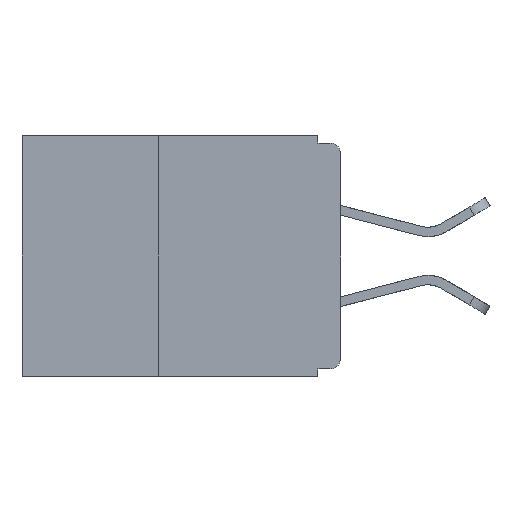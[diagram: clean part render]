
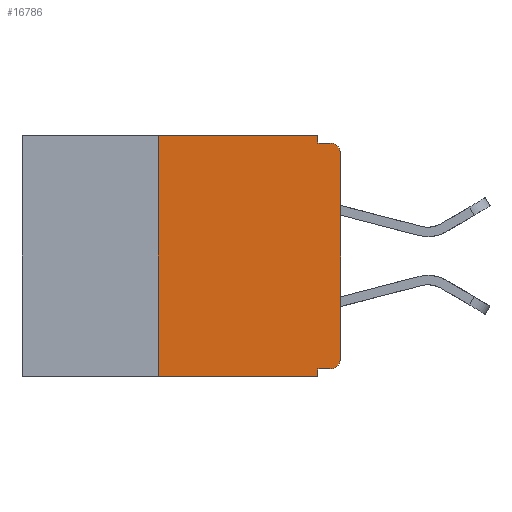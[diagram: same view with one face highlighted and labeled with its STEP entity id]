
A CAD part, left-side view. The second image highlights one B-rep face of the part: STEP entity #16786.
In plain terms, the highlighted planar face has unit normal (-1, 0, 0).
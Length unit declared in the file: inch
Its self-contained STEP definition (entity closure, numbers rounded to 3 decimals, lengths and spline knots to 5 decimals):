
#333 = EDGE_CURVE ( 'NONE', #7739, #5387, #16502, .T. ) ;
#369 = EDGE_CURVE ( 'NONE', #20299, #21853, #20265, .T. ) ;
#513 = ORIENTED_EDGE ( 'NONE', *, *, #4288, .T. ) ;
#768 = EDGE_CURVE ( 'NONE', #16155, #20713, #16186, .T. ) ;
#907 = FACE_OUTER_BOUND ( 'NONE', #26456, .T. ) ;
#1850 = EDGE_CURVE ( 'NONE', #24167, #23509, #6395, .T. ) ;
#2306 = LINE ( 'NONE', #22788, #8103 ) ;
#2898 = ORIENTED_EDGE ( 'NONE', *, *, #369, .F. ) ;
#3325 = AXIS2_PLACEMENT_3D ( 'NONE', #27504, #6271, #21327 ) ;
#3384 = VERTEX_POINT ( 'NONE', #24861 ) ;
#3418 = VECTOR ( 'NONE', #6739, 39.37008 ) ;
#3450 = EDGE_CURVE ( 'NONE', #23509, #7739, #2306, .T. ) ;
#4116 = CARTESIAN_POINT ( 'NONE',  ( 0., 0.031, 0. ) ) ;
#4288 = EDGE_CURVE ( 'NONE', #16155, #3384, #4691, .T. ) ;
#4626 = ORIENTED_EDGE ( 'NONE', *, *, #19297, .F. ) ;
#4691 = LINE ( 'NONE', #25082, #14783 ) ;
#4969 = LINE ( 'NONE', #11244, #21479 ) ;
#5387 = VERTEX_POINT ( 'NONE', #11502 ) ;
#6271 = DIRECTION ( 'NONE',  ( 1., 0., 0. ) ) ;
#6303 = CARTESIAN_POINT ( 'NONE',  ( 0., 0.25, -0.33 ) ) ;
#6395 = CIRCLE ( 'NONE', #24870, 0.015 ) ;
#6739 = DIRECTION ( 'NONE',  ( 0., 0., -1. ) ) ;
#7111 = EDGE_CURVE ( 'NONE', #21853, #5387, #20381, .T. ) ;
#7495 = CARTESIAN_POINT ( 'NONE',  ( 0., 0.25, -0.33 ) ) ;
#7684 = DIRECTION ( 'NONE',  ( -1., 0., 0. ) ) ;
#7739 = VERTEX_POINT ( 'NONE', #9589 ) ;
#7931 = CARTESIAN_POINT ( 'NONE',  ( 0., 0.015, -0.305 ) ) ;
#8103 = VECTOR ( 'NONE', #22433, 39.37008 ) ;
#8962 = VECTOR ( 'NONE', #20363, 39.37008 ) ;
#9033 = DIRECTION ( 'NONE',  ( 0., 0., -1. ) ) ;
#9088 = CARTESIAN_POINT ( 'NONE',  ( 0., 0.015, -0.32 ) ) ;
#9246 = EDGE_CURVE ( 'NONE', #26113, #3384, #22892, .T. ) ;
#9589 = CARTESIAN_POINT ( 'NONE',  ( 0., 0., -0.025 ) ) ;
#9599 = DIRECTION ( 'NONE',  ( 0., 1., 0. ) ) ;
#10037 = ORIENTED_EDGE ( 'NONE', *, *, #768, .F. ) ;
#10521 = DIRECTION ( 'NONE',  ( 0., 0., 1. ) ) ;
#11244 = CARTESIAN_POINT ( 'NONE',  ( 0., 0.437, 0. ) ) ;
#11502 = CARTESIAN_POINT ( 'NONE',  ( 0., 0.015, -0.01 ) ) ;
#11732 = ORIENTED_EDGE ( 'NONE', *, *, #333, .T. ) ;
#12503 = CARTESIAN_POINT ( 'NONE',  ( 0., 0.031, -0.33 ) ) ;
#12570 = DIRECTION ( 'NONE',  ( 0., 0., -1. ) ) ;
#12828 = CARTESIAN_POINT ( 'NONE',  ( 0., 0.031, -0.32 ) ) ;
#14371 = ORIENTED_EDGE ( 'NONE', *, *, #24363, .F. ) ;
#14783 = VECTOR ( 'NONE', #25294, 39.37008 ) ;
#15270 = VECTOR ( 'NONE', #9599, 39.37008 ) ;
#15272 = CARTESIAN_POINT ( 'NONE',  ( 0., 0., -0.305 ) ) ;
#15934 = CARTESIAN_POINT ( 'NONE',  ( 0., 0., -0.32 ) ) ;
#16155 = VERTEX_POINT ( 'NONE', #6303 ) ;
#16186 = LINE ( 'NONE', #7495, #26834 ) ;
#16502 = CIRCLE ( 'NONE', #20468, 0.015 ) ;
#16725 = ORIENTED_EDGE ( 'NONE', *, *, #1850, .T. ) ;
#16786 = ADVANCED_FACE ( 'NONE', ( #907 ), #19172, .F. ) ;
#17716 = CARTESIAN_POINT ( 'NONE',  ( 0., 0.031, -0.01 ) ) ;
#17889 = VECTOR ( 'NONE', #12570, 39.37008 ) ;
#19123 = ORIENTED_EDGE ( 'NONE', *, *, #9246, .F. ) ;
#19172 = PLANE ( 'NONE',  #3325 ) ;
#19297 = EDGE_CURVE ( 'NONE', #24167, #26113, #21018, .T. ) ;
#19457 = ORIENTED_EDGE ( 'NONE', *, *, #7111, .F. ) ;
#20241 = CARTESIAN_POINT ( 'NONE',  ( 0., 0., -0.01 ) ) ;
#20265 = LINE ( 'NONE', #4116, #3418 ) ;
#20299 = VERTEX_POINT ( 'NONE', #25571 ) ;
#20363 = DIRECTION ( 'NONE',  ( 0., -1., 0. ) ) ;
#20381 = LINE ( 'NONE', #20241, #8962 ) ;
#20468 = AXIS2_PLACEMENT_3D ( 'NONE', #21932, #22123, #27220 ) ;
#20713 = VERTEX_POINT ( 'NONE', #22734 ) ;
#21018 = LINE ( 'NONE', #15934, #15270 ) ;
#21327 = DIRECTION ( 'NONE',  ( 0., 0., -1. ) ) ;
#21479 = VECTOR ( 'NONE', #24029, 39.37008 ) ;
#21790 = ORIENTED_EDGE ( 'NONE', *, *, #3450, .T. ) ;
#21853 = VERTEX_POINT ( 'NONE', #17716 ) ;
#21932 = CARTESIAN_POINT ( 'NONE',  ( 0., 0.015, -0.025 ) ) ;
#22123 = DIRECTION ( 'NONE',  ( -1., 0., 0. ) ) ;
#22433 = DIRECTION ( 'NONE',  ( 0., 0., 1. ) ) ;
#22734 = CARTESIAN_POINT ( 'NONE',  ( 0., 0.25, 0. ) ) ;
#22788 = CARTESIAN_POINT ( 'NONE',  ( 0., 0., 0. ) ) ;
#22892 = LINE ( 'NONE', #12503, #17889 ) ;
#23509 = VERTEX_POINT ( 'NONE', #15272 ) ;
#24029 = DIRECTION ( 'NONE',  ( 0., -1., 0. ) ) ;
#24167 = VERTEX_POINT ( 'NONE', #9088 ) ;
#24363 = EDGE_CURVE ( 'NONE', #20713, #20299, #4969, .T. ) ;
#24861 = CARTESIAN_POINT ( 'NONE',  ( 0., 0.031, -0.33 ) ) ;
#24870 = AXIS2_PLACEMENT_3D ( 'NONE', #7931, #7684, #9033 ) ;
#25082 = CARTESIAN_POINT ( 'NONE',  ( 0., 0.437, -0.33 ) ) ;
#25294 = DIRECTION ( 'NONE',  ( 0., -1., 0. ) ) ;
#25571 = CARTESIAN_POINT ( 'NONE',  ( 0., 0.031, 0. ) ) ;
#26113 = VERTEX_POINT ( 'NONE', #12828 ) ;
#26456 = EDGE_LOOP ( 'NONE', ( #21790, #11732, #19457, #2898, #14371, #10037, #513, #19123, #4626, #16725 ) ) ;
#26834 = VECTOR ( 'NONE', #10521, 39.37008 ) ;
#27220 = DIRECTION ( 'NONE',  ( 0., 0., -1. ) ) ;
#27504 = CARTESIAN_POINT ( 'NONE',  ( 0., 0.437, 0. ) ) ;
